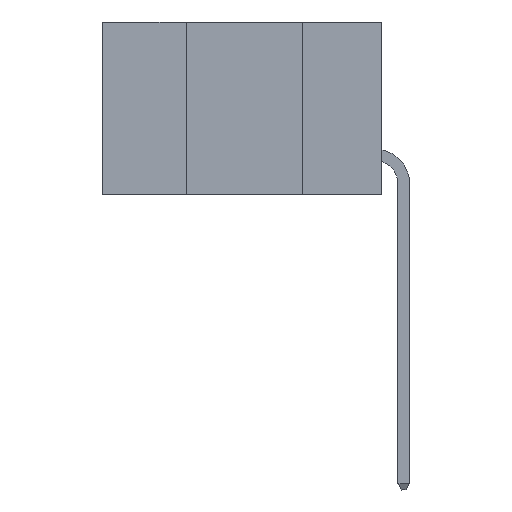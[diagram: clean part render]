
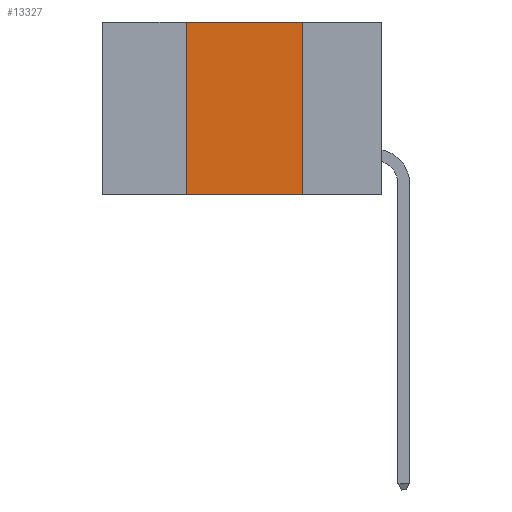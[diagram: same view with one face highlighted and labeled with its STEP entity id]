
A CAD part, left-side view. The second image highlights one B-rep face of the part: STEP entity #13327.
In plain terms, the highlighted planar face has unit normal (-1, 0, 0).
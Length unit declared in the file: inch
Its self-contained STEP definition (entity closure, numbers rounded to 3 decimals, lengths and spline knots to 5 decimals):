
#1189 = LINE ( 'NONE', #20210, #22609 ) ;
#1717 = CARTESIAN_POINT ( 'NONE',  ( 0., 0.42, 0. ) ) ;
#2338 = PLANE ( 'NONE',  #9315 ) ;
#2903 = LINE ( 'NONE', #22221, #23006 ) ;
#2992 = DIRECTION ( 'NONE',  ( 0., -1., 0. ) ) ;
#3551 = CARTESIAN_POINT ( 'NONE',  ( 0., 0.42, 0. ) ) ;
#4429 = EDGE_CURVE ( 'NONE', #24547, #5541, #16948, .T. ) ;
#4538 = DIRECTION ( 'NONE',  ( 1., 0., 0. ) ) ;
#5541 = VERTEX_POINT ( 'NONE', #5569 ) ;
#5569 = CARTESIAN_POINT ( 'NONE',  ( 0., 0.17, 0. ) ) ;
#5602 = EDGE_CURVE ( 'NONE', #15758, #23379, #2903, .T. ) ;
#7446 = ORIENTED_EDGE ( 'NONE', *, *, #11155, .F. ) ;
#8971 = VECTOR ( 'NONE', #18316, 39.37008 ) ;
#9315 = AXIS2_PLACEMENT_3D ( 'NONE', #12829, #4538, #19031 ) ;
#9342 = ORIENTED_EDGE ( 'NONE', *, *, #4429, .F. ) ;
#9783 = EDGE_CURVE ( 'NONE', #5541, #23379, #1189, .T. ) ;
#9812 = DIRECTION ( 'NONE',  ( 0., 0., -1. ) ) ;
#10129 = FACE_OUTER_BOUND ( 'NONE', #20953, .T. ) ;
#11155 = EDGE_CURVE ( 'NONE', #15758, #24547, #15107, .T. ) ;
#12262 = CARTESIAN_POINT ( 'NONE',  ( 0., 0.17, -0.37 ) ) ;
#12279 = ORIENTED_EDGE ( 'NONE', *, *, #9783, .F. ) ;
#12829 = CARTESIAN_POINT ( 'NONE',  ( 0., 0.6, 0. ) ) ;
#13327 = ADVANCED_FACE ( 'NONE', ( #10129 ), #2338, .F. ) ;
#15107 = LINE ( 'NONE', #1717, #8971 ) ;
#15758 = VERTEX_POINT ( 'NONE', #20415 ) ;
#16087 = DIRECTION ( 'NONE',  ( 0., -1., 0. ) ) ;
#16948 = LINE ( 'NONE', #21578, #25922 ) ;
#18316 = DIRECTION ( 'NONE',  ( 0., 0., 1. ) ) ;
#19031 = DIRECTION ( 'NONE',  ( 0., 0., -1. ) ) ;
#19713 = ORIENTED_EDGE ( 'NONE', *, *, #5602, .T. ) ;
#20210 = CARTESIAN_POINT ( 'NONE',  ( 0., 0.17, 0. ) ) ;
#20415 = CARTESIAN_POINT ( 'NONE',  ( 0., 0.42, -0.37 ) ) ;
#20953 = EDGE_LOOP ( 'NONE', ( #12279, #9342, #7446, #19713 ) ) ;
#21578 = CARTESIAN_POINT ( 'NONE',  ( 0., 0.6, 0. ) ) ;
#22221 = CARTESIAN_POINT ( 'NONE',  ( 0., 0.6, -0.37 ) ) ;
#22609 = VECTOR ( 'NONE', #9812, 39.37008 ) ;
#23006 = VECTOR ( 'NONE', #16087, 39.37008 ) ;
#23379 = VERTEX_POINT ( 'NONE', #12262 ) ;
#24547 = VERTEX_POINT ( 'NONE', #3551 ) ;
#25922 = VECTOR ( 'NONE', #2992, 39.37008 ) ;
